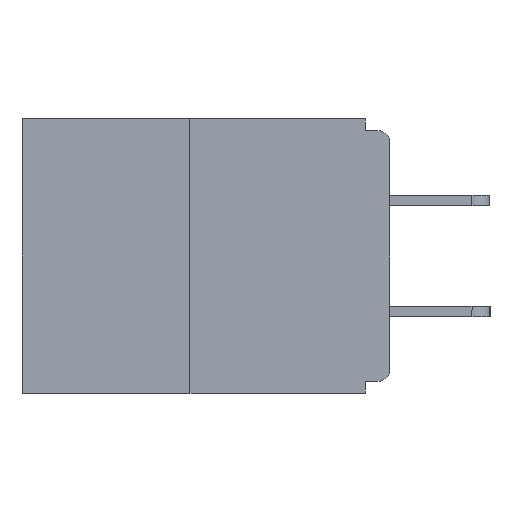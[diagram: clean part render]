
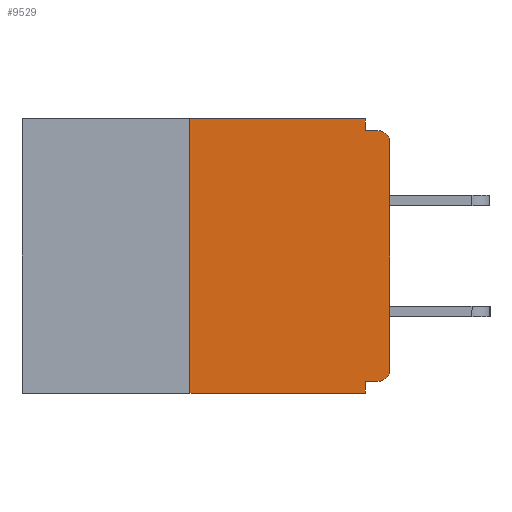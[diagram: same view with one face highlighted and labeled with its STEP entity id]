
A CAD part, left-side view. The second image highlights one B-rep face of the part: STEP entity #9529.
In plain terms, the highlighted planar face has unit normal (-1, 0, 0).
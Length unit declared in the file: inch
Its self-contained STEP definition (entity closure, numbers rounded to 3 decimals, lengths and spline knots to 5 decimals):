
#13 = PLANE ( 'NONE',  #20649 ) ;
#353 = DIRECTION ( 'NONE',  ( 0., 0., -1. ) ) ;
#580 = VECTOR ( 'NONE', #8269, 39.37008 ) ;
#1245 = EDGE_CURVE ( 'NONE', #13603, #1577, #12945, .T. ) ;
#1577 = VERTEX_POINT ( 'NONE', #9364 ) ;
#1789 = CARTESIAN_POINT ( 'NONE',  ( 0., 0.031, -0.343 ) ) ;
#2490 = CARTESIAN_POINT ( 'NONE',  ( 0., 0.25, 0. ) ) ;
#3058 = FACE_OUTER_BOUND ( 'NONE', #16466, .T. ) ;
#3384 = VECTOR ( 'NONE', #23274, 39.37008 ) ;
#3619 = LINE ( 'NONE', #27159, #14444 ) ;
#4022 = EDGE_CURVE ( 'NONE', #22625, #26315, #21959, .T. ) ;
#4242 = DIRECTION ( 'NONE',  ( 0., 0., -1. ) ) ;
#4318 = DIRECTION ( 'NONE',  ( 0., 0., 1. ) ) ;
#4413 = EDGE_CURVE ( 'NONE', #21176, #24396, #3619, .T. ) ;
#5118 = DIRECTION ( 'NONE',  ( 0., -1., 0. ) ) ;
#5943 = VECTOR ( 'NONE', #21823, 39.37008 ) ;
#6036 = DIRECTION ( 'NONE',  ( -1., 0., 0. ) ) ;
#6149 = CARTESIAN_POINT ( 'NONE',  ( 0., 0.031, -0.015 ) ) ;
#6742 = CIRCLE ( 'NONE', #16022, 0.015 ) ;
#6806 = VECTOR ( 'NONE', #4318, 39.37008 ) ;
#7400 = ORIENTED_EDGE ( 'NONE', *, *, #1245, .F. ) ;
#7604 = CARTESIAN_POINT ( 'NONE',  ( 0., 0., 0. ) ) ;
#7616 = LINE ( 'NONE', #13344, #14032 ) ;
#7798 = CARTESIAN_POINT ( 'NONE',  ( 0., 0., -0.313 ) ) ;
#8033 = DIRECTION ( 'NONE',  ( 0., 0., -1. ) ) ;
#8269 = DIRECTION ( 'NONE',  ( 0., -1., 0. ) ) ;
#8486 = LINE ( 'NONE', #2490, #6806 ) ;
#8640 = DIRECTION ( 'NONE',  ( 1., 0., 0. ) ) ;
#8838 = EDGE_CURVE ( 'NONE', #26315, #13603, #9203, .T. ) ;
#9203 = LINE ( 'NONE', #23293, #25816 ) ;
#9362 = EDGE_CURVE ( 'NONE', #20038, #22625, #8486, .T. ) ;
#9364 = CARTESIAN_POINT ( 'NONE',  ( 0., 0.015, -0.015 ) ) ;
#9529 = ADVANCED_FACE ( 'NONE', ( #3058 ), #13, .F. ) ;
#9839 = LINE ( 'NONE', #14426, #3384 ) ;
#10016 = CARTESIAN_POINT ( 'NONE',  ( 0., 0.25, -0.343 ) ) ;
#10943 = VERTEX_POINT ( 'NONE', #21985 ) ;
#11798 = ORIENTED_EDGE ( 'NONE', *, *, #4022, .F. ) ;
#11985 = ORIENTED_EDGE ( 'NONE', *, *, #14219, .F. ) ;
#12945 = LINE ( 'NONE', #19040, #25828 ) ;
#13031 = ORIENTED_EDGE ( 'NONE', *, *, #27373, .T. ) ;
#13344 = CARTESIAN_POINT ( 'NONE',  ( 0., 0.46, -0.343 ) ) ;
#13603 = VERTEX_POINT ( 'NONE', #6149 ) ;
#14032 = VECTOR ( 'NONE', #5118, 39.37008 ) ;
#14058 = DIRECTION ( 'NONE',  ( -1., 0., 0. ) ) ;
#14219 = EDGE_CURVE ( 'NONE', #20239, #21176, #9839, .T. ) ;
#14426 = CARTESIAN_POINT ( 'NONE',  ( 0., 0., -0.328 ) ) ;
#14444 = VECTOR ( 'NONE', #25087, 39.37008 ) ;
#14576 = DIRECTION ( 'NONE',  ( 0., -1., 0. ) ) ;
#15144 = DIRECTION ( 'NONE',  ( 0., 0., -1. ) ) ;
#15206 = CARTESIAN_POINT ( 'NONE',  ( 0., 0.015, -0.328 ) ) ;
#15232 = ORIENTED_EDGE ( 'NONE', *, *, #4413, .F. ) ;
#15505 = CARTESIAN_POINT ( 'NONE',  ( 0., 0.015, -0.313 ) ) ;
#16022 = AXIS2_PLACEMENT_3D ( 'NONE', #15505, #14058, #353 ) ;
#16466 = EDGE_LOOP ( 'NONE', ( #11798, #27247, #27421, #15232, #11985, #26724, #21910, #13031, #7400, #17738 ) ) ;
#17678 = EDGE_CURVE ( 'NONE', #18057, #10943, #21179, .T. ) ;
#17738 = ORIENTED_EDGE ( 'NONE', *, *, #8838, .F. ) ;
#18057 = VERTEX_POINT ( 'NONE', #7798 ) ;
#19040 = CARTESIAN_POINT ( 'NONE',  ( 0., 0., -0.015 ) ) ;
#19220 = CARTESIAN_POINT ( 'NONE',  ( 0., 0.46, 0. ) ) ;
#19564 = CARTESIAN_POINT ( 'NONE',  ( 0., 0.031, 0. ) ) ;
#20038 = VERTEX_POINT ( 'NONE', #10016 ) ;
#20239 = VERTEX_POINT ( 'NONE', #15206 ) ;
#20649 = AXIS2_PLACEMENT_3D ( 'NONE', #19220, #8640, #15144 ) ;
#21161 = CIRCLE ( 'NONE', #23916, 0.015 ) ;
#21176 = VERTEX_POINT ( 'NONE', #21649 ) ;
#21179 = LINE ( 'NONE', #7604, #5943 ) ;
#21649 = CARTESIAN_POINT ( 'NONE',  ( 0., 0.031, -0.328 ) ) ;
#21823 = DIRECTION ( 'NONE',  ( 0., 0., 1. ) ) ;
#21910 = ORIENTED_EDGE ( 'NONE', *, *, #17678, .T. ) ;
#21959 = LINE ( 'NONE', #23152, #580 ) ;
#21985 = CARTESIAN_POINT ( 'NONE',  ( 0., 0., -0.03 ) ) ;
#22625 = VERTEX_POINT ( 'NONE', #26055 ) ;
#23152 = CARTESIAN_POINT ( 'NONE',  ( 0., 0.46, 0. ) ) ;
#23274 = DIRECTION ( 'NONE',  ( 0., 1., 0. ) ) ;
#23293 = CARTESIAN_POINT ( 'NONE',  ( 0., 0.031, 0. ) ) ;
#23916 = AXIS2_PLACEMENT_3D ( 'NONE', #25821, #6036, #4242 ) ;
#24396 = VERTEX_POINT ( 'NONE', #1789 ) ;
#25087 = DIRECTION ( 'NONE',  ( 0., 0., -1. ) ) ;
#25090 = EDGE_CURVE ( 'NONE', #20239, #18057, #6742, .T. ) ;
#25816 = VECTOR ( 'NONE', #8033, 39.37008 ) ;
#25821 = CARTESIAN_POINT ( 'NONE',  ( 0., 0.015, -0.03 ) ) ;
#25828 = VECTOR ( 'NONE', #14576, 39.37008 ) ;
#26055 = CARTESIAN_POINT ( 'NONE',  ( 0., 0.25, 0. ) ) ;
#26315 = VERTEX_POINT ( 'NONE', #19564 ) ;
#26724 = ORIENTED_EDGE ( 'NONE', *, *, #25090, .T. ) ;
#27097 = EDGE_CURVE ( 'NONE', #20038, #24396, #7616, .T. ) ;
#27159 = CARTESIAN_POINT ( 'NONE',  ( 0., 0.031, -0.343 ) ) ;
#27247 = ORIENTED_EDGE ( 'NONE', *, *, #9362, .F. ) ;
#27373 = EDGE_CURVE ( 'NONE', #10943, #1577, #21161, .T. ) ;
#27421 = ORIENTED_EDGE ( 'NONE', *, *, #27097, .T. ) ;
